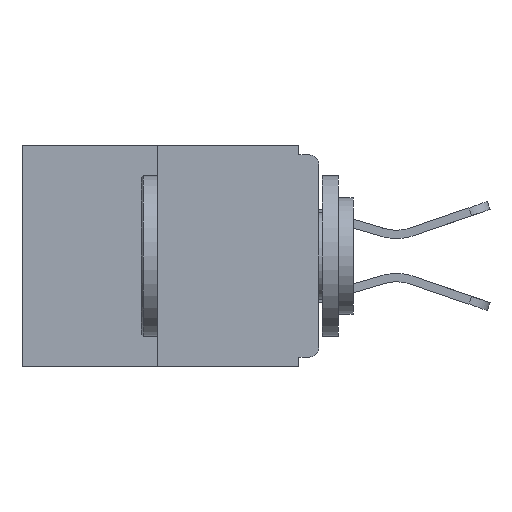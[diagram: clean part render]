
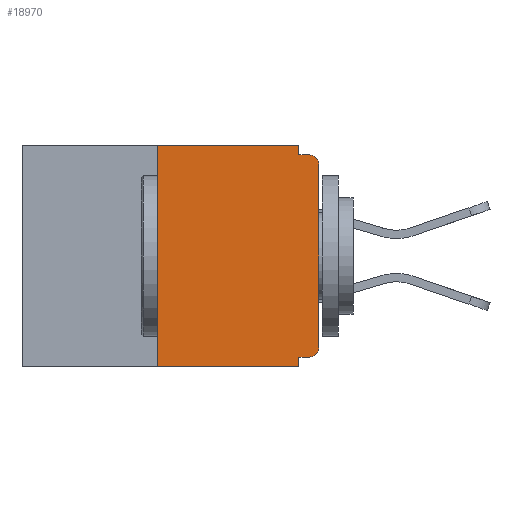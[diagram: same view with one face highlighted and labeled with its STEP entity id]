
A CAD part, left-side view. The second image highlights one B-rep face of the part: STEP entity #18970.
In plain terms, the highlighted planar face has unit normal (-1, 0, 0).
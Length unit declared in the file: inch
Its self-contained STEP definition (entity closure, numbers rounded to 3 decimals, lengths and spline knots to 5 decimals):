
#339 = EDGE_CURVE ( 'NONE', #1532, #9076, #12816, .T. ) ;
#959 = AXIS2_PLACEMENT_3D ( 'NONE', #14375, #3218, #10979 ) ;
#1154 = ORIENTED_EDGE ( 'NONE', *, *, #2205, .T. ) ;
#1271 = VERTEX_POINT ( 'NONE', #9269 ) ;
#1457 = VECTOR ( 'NONE', #6376, 39.37008 ) ;
#1532 = VERTEX_POINT ( 'NONE', #12883 ) ;
#1893 = DIRECTION ( 'NONE',  ( 0., -1., 0. ) ) ;
#1921 = ORIENTED_EDGE ( 'NONE', *, *, #20461, .T. ) ;
#2205 = EDGE_CURVE ( 'NONE', #1532, #14384, #10853, .T. ) ;
#3218 = DIRECTION ( 'NONE',  ( -1., 0., 0. ) ) ;
#3407 = EDGE_CURVE ( 'NONE', #20767, #1271, #4943, .T. ) ;
#3432 = AXIS2_PLACEMENT_3D ( 'NONE', #18020, #16140, #12655 ) ;
#3790 = ORIENTED_EDGE ( 'NONE', *, *, #9330, .F. ) ;
#4080 = ORIENTED_EDGE ( 'NONE', *, *, #12907, .T. ) ;
#4134 = CARTESIAN_POINT ( 'NONE',  ( 0., 0.46, 0. ) ) ;
#4140 = CARTESIAN_POINT ( 'NONE',  ( 0., 0.031, -0.343 ) ) ;
#4165 = ORIENTED_EDGE ( 'NONE', *, *, #339, .F. ) ;
#4616 = CARTESIAN_POINT ( 'NONE',  ( 0., 0.031, 0. ) ) ;
#4943 = LINE ( 'NONE', #13341, #5828 ) ;
#5828 = VECTOR ( 'NONE', #5901, 39.37008 ) ;
#5901 = DIRECTION ( 'NONE',  ( 0., -1., 0. ) ) ;
#6101 = CARTESIAN_POINT ( 'NONE',  ( 0., 0.031, -0.015 ) ) ;
#6376 = DIRECTION ( 'NONE',  ( 0., 0., 1. ) ) ;
#6813 = VECTOR ( 'NONE', #16842, 39.37008 ) ;
#7299 = CARTESIAN_POINT ( 'NONE',  ( 0., 0.031, 0. ) ) ;
#7301 = AXIS2_PLACEMENT_3D ( 'NONE', #17208, #19092, #9755 ) ;
#7582 = ORIENTED_EDGE ( 'NONE', *, *, #3407, .F. ) ;
#9076 = VERTEX_POINT ( 'NONE', #23422 ) ;
#9193 = LINE ( 'NONE', #4140, #6813 ) ;
#9269 = CARTESIAN_POINT ( 'NONE',  ( 0., 0.015, -0.015 ) ) ;
#9330 = EDGE_CURVE ( 'NONE', #16863, #14384, #9193, .T. ) ;
#9729 = FACE_OUTER_BOUND ( 'NONE', #17043, .T. ) ;
#9755 = DIRECTION ( 'NONE',  ( 0., 0., -1. ) ) ;
#9757 = LINE ( 'NONE', #7299, #20504 ) ;
#9908 = CIRCLE ( 'NONE', #7301, 0.015 ) ;
#9936 = DIRECTION ( 'NONE',  ( 0., 0., 1. ) ) ;
#10803 = EDGE_CURVE ( 'NONE', #11809, #20767, #9757, .T. ) ;
#10853 = LINE ( 'NONE', #11278, #23656 ) ;
#10979 = DIRECTION ( 'NONE',  ( 0., 0., -1. ) ) ;
#11278 = CARTESIAN_POINT ( 'NONE',  ( 0., 0.46, -0.343 ) ) ;
#11328 = CARTESIAN_POINT ( 'NONE',  ( 0., 0.25, 0. ) ) ;
#11580 = CARTESIAN_POINT ( 'NONE',  ( 0., 0., -0.328 ) ) ;
#11809 = VERTEX_POINT ( 'NONE', #4616 ) ;
#12655 = DIRECTION ( 'NONE',  ( 0., 0., -1. ) ) ;
#12816 = LINE ( 'NONE', #11328, #17190 ) ;
#12883 = CARTESIAN_POINT ( 'NONE',  ( 0., 0.25, -0.343 ) ) ;
#12907 = EDGE_CURVE ( 'NONE', #23094, #23750, #9908, .T. ) ;
#13341 = CARTESIAN_POINT ( 'NONE',  ( 0., 0., -0.015 ) ) ;
#13345 = VECTOR ( 'NONE', #20919, 39.37008 ) ;
#13790 = CARTESIAN_POINT ( 'NONE',  ( 0., 0.015, -0.328 ) ) ;
#13923 = ORIENTED_EDGE ( 'NONE', *, *, #10803, .F. ) ;
#14375 = CARTESIAN_POINT ( 'NONE',  ( 0., 0.015, -0.03 ) ) ;
#14384 = VERTEX_POINT ( 'NONE', #14993 ) ;
#14618 = LINE ( 'NONE', #11580, #23935 ) ;
#14627 = CARTESIAN_POINT ( 'NONE',  ( 0., 0., -0.313 ) ) ;
#14898 = LINE ( 'NONE', #19200, #1457 ) ;
#14993 = CARTESIAN_POINT ( 'NONE',  ( 0., 0.031, -0.343 ) ) ;
#15752 = EDGE_CURVE ( 'NONE', #9076, #11809, #22328, .T. ) ;
#16140 = DIRECTION ( 'NONE',  ( 1., 0., 0. ) ) ;
#16842 = DIRECTION ( 'NONE',  ( 0., 0., -1. ) ) ;
#16863 = VERTEX_POINT ( 'NONE', #19862 ) ;
#17043 = EDGE_LOOP ( 'NONE', ( #23470, #4165, #1154, #3790, #17249, #4080, #1921, #19961, #7582, #13923 ) ) ;
#17190 = VECTOR ( 'NONE', #9936, 39.37008 ) ;
#17208 = CARTESIAN_POINT ( 'NONE',  ( 0., 0.015, -0.313 ) ) ;
#17249 = ORIENTED_EDGE ( 'NONE', *, *, #19236, .F. ) ;
#18020 = CARTESIAN_POINT ( 'NONE',  ( 0., 0.46, 0. ) ) ;
#18067 = CARTESIAN_POINT ( 'NONE',  ( 0., 0., -0.03 ) ) ;
#18354 = CIRCLE ( 'NONE', #959, 0.015 ) ;
#18970 = ADVANCED_FACE ( 'NONE', ( #9729 ), #23547, .F. ) ;
#19092 = DIRECTION ( 'NONE',  ( -1., 0., 0. ) ) ;
#19200 = CARTESIAN_POINT ( 'NONE',  ( 0., 0., 0. ) ) ;
#19236 = EDGE_CURVE ( 'NONE', #23094, #16863, #14618, .T. ) ;
#19862 = CARTESIAN_POINT ( 'NONE',  ( 0., 0.031, -0.328 ) ) ;
#19961 = ORIENTED_EDGE ( 'NONE', *, *, #21217, .T. ) ;
#20461 = EDGE_CURVE ( 'NONE', #23750, #23477, #14898, .T. ) ;
#20504 = VECTOR ( 'NONE', #22275, 39.37008 ) ;
#20675 = DIRECTION ( 'NONE',  ( 0., 1., 0. ) ) ;
#20767 = VERTEX_POINT ( 'NONE', #6101 ) ;
#20919 = DIRECTION ( 'NONE',  ( 0., -1., 0. ) ) ;
#21217 = EDGE_CURVE ( 'NONE', #23477, #1271, #18354, .T. ) ;
#22275 = DIRECTION ( 'NONE',  ( 0., 0., -1. ) ) ;
#22328 = LINE ( 'NONE', #4134, #13345 ) ;
#23094 = VERTEX_POINT ( 'NONE', #13790 ) ;
#23422 = CARTESIAN_POINT ( 'NONE',  ( 0., 0.25, 0. ) ) ;
#23470 = ORIENTED_EDGE ( 'NONE', *, *, #15752, .F. ) ;
#23477 = VERTEX_POINT ( 'NONE', #18067 ) ;
#23547 = PLANE ( 'NONE',  #3432 ) ;
#23656 = VECTOR ( 'NONE', #1893, 39.37008 ) ;
#23750 = VERTEX_POINT ( 'NONE', #14627 ) ;
#23935 = VECTOR ( 'NONE', #20675, 39.37008 ) ;
